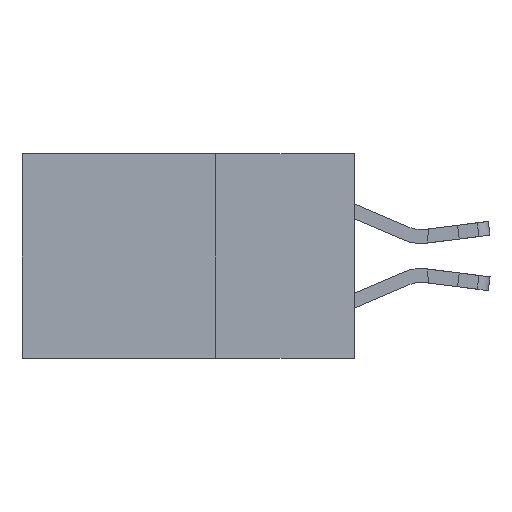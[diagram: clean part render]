
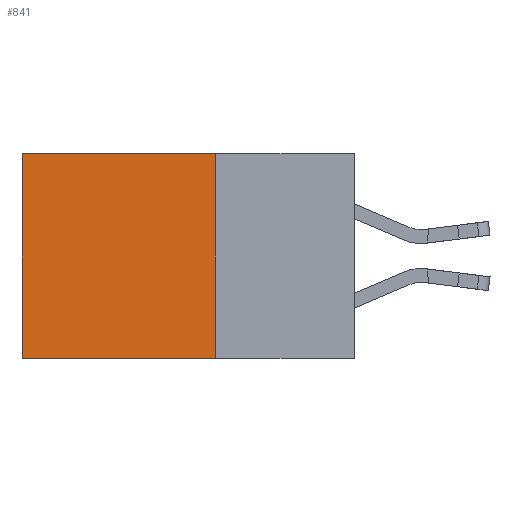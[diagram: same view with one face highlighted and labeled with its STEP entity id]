
A CAD part, left-side view. The second image highlights one B-rep face of the part: STEP entity #841.
In plain terms, the highlighted planar face has unit normal (-1, 0, 0).
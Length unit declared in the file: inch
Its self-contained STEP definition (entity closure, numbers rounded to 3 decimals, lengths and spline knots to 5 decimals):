
#659 = CARTESIAN_POINT ( 'NONE',  ( 0.2615, 0.25, 0. ) ) ;
#841 = ADVANCED_FACE ( 'NONE', ( #20405 ), #2747, .F. ) ;
#1171 = CARTESIAN_POINT ( 'NONE',  ( 0.2615, 0.25, -0.37 ) ) ;
#1598 = EDGE_LOOP ( 'NONE', ( #20890, #4578, #6670, #12532 ) ) ;
#2001 = DIRECTION ( 'NONE',  ( 0., 0., -1. ) ) ;
#2747 = PLANE ( 'NONE',  #9788 ) ;
#3733 = EDGE_CURVE ( 'NONE', #20516, #13512, #8931, .T. ) ;
#4578 = ORIENTED_EDGE ( 'NONE', *, *, #19994, .F. ) ;
#5020 = VERTEX_POINT ( 'NONE', #17914 ) ;
#6105 = EDGE_CURVE ( 'NONE', #20516, #7185, #13087, .T. ) ;
#6670 = ORIENTED_EDGE ( 'NONE', *, *, #3733, .F. ) ;
#7018 = CARTESIAN_POINT ( 'NONE',  ( 0.2615, 0.25, -0.37 ) ) ;
#7185 = VERTEX_POINT ( 'NONE', #12296 ) ;
#7217 = LINE ( 'NONE', #13824, #20896 ) ;
#8176 = CARTESIAN_POINT ( 'NONE',  ( 0.2615, 0.25, 0. ) ) ;
#8716 = VECTOR ( 'NONE', #12963, 39.37008 ) ;
#8931 = LINE ( 'NONE', #7018, #18254 ) ;
#9788 = AXIS2_PLACEMENT_3D ( 'NONE', #16851, #18637, #15809 ) ;
#11542 = DIRECTION ( 'NONE',  ( 0., 1., 0. ) ) ;
#12296 = CARTESIAN_POINT ( 'NONE',  ( 0.2615, 0.6, 0. ) ) ;
#12532 = ORIENTED_EDGE ( 'NONE', *, *, #6105, .T. ) ;
#12963 = DIRECTION ( 'NONE',  ( 0., 1., 0. ) ) ;
#13087 = LINE ( 'NONE', #8176, #17481 ) ;
#13117 = LINE ( 'NONE', #17880, #8716 ) ;
#13512 = VERTEX_POINT ( 'NONE', #1171 ) ;
#13824 = CARTESIAN_POINT ( 'NONE',  ( 0.2615, 0.6, -0.37 ) ) ;
#13856 = EDGE_CURVE ( 'NONE', #7185, #5020, #7217, .T. ) ;
#15809 = DIRECTION ( 'NONE',  ( 0., 0., -1. ) ) ;
#16821 = DIRECTION ( 'NONE',  ( 0., 0., -1. ) ) ;
#16851 = CARTESIAN_POINT ( 'NONE',  ( 0.2615, 0.25, -0.37 ) ) ;
#17481 = VECTOR ( 'NONE', #11542, 39.37008 ) ;
#17880 = CARTESIAN_POINT ( 'NONE',  ( 0.2615, 0.25, -0.37 ) ) ;
#17914 = CARTESIAN_POINT ( 'NONE',  ( 0.2615, 0.6, -0.37 ) ) ;
#18254 = VECTOR ( 'NONE', #16821, 39.37008 ) ;
#18637 = DIRECTION ( 'NONE',  ( 1., 0., 0. ) ) ;
#19994 = EDGE_CURVE ( 'NONE', #13512, #5020, #13117, .T. ) ;
#20405 = FACE_OUTER_BOUND ( 'NONE', #1598, .T. ) ;
#20516 = VERTEX_POINT ( 'NONE', #659 ) ;
#20890 = ORIENTED_EDGE ( 'NONE', *, *, #13856, .T. ) ;
#20896 = VECTOR ( 'NONE', #2001, 39.37008 ) ;
